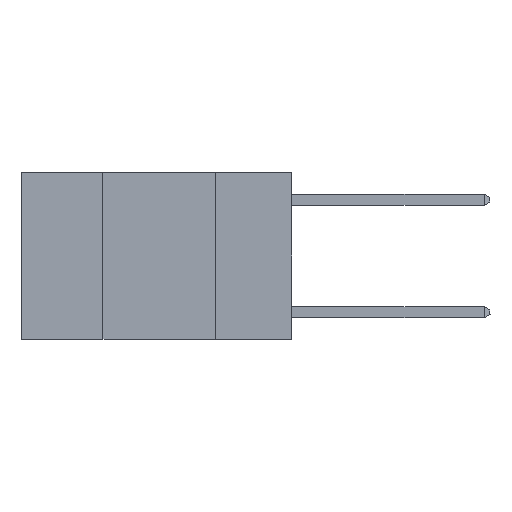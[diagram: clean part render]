
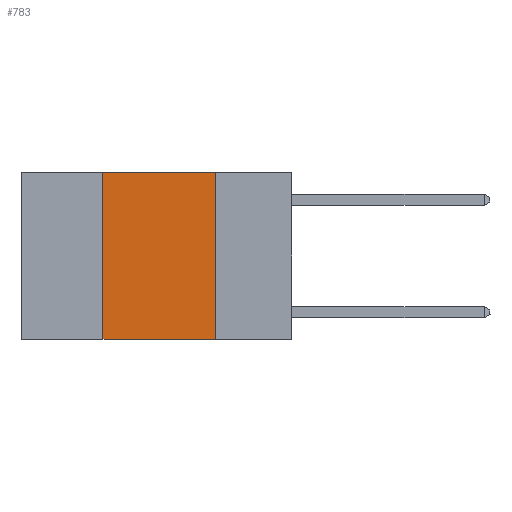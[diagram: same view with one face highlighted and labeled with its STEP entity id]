
A CAD part, left-side view. The second image highlights one B-rep face of the part: STEP entity #783.
In plain terms, the highlighted planar face has unit normal (-1, 0, 0).
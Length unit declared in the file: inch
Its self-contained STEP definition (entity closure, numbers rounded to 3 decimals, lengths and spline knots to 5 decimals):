
#232 = LINE ( 'NONE', #2339, #8810 ) ;
#305 = CARTESIAN_POINT ( 'NONE',  ( 0., 0.6, 0. ) ) ;
#434 = FACE_OUTER_BOUND ( 'NONE', #3041, .T. ) ;
#455 = VERTEX_POINT ( 'NONE', #8844 ) ;
#783 = ADVANCED_FACE ( 'NONE', ( #434 ), #3638, .F. ) ;
#1114 = ORIENTED_EDGE ( 'NONE', *, *, #6285, .F. ) ;
#1463 = ORIENTED_EDGE ( 'NONE', *, *, #6756, .F. ) ;
#1543 = DIRECTION ( 'NONE',  ( 0., 0., 1. ) ) ;
#1560 = VERTEX_POINT ( 'NONE', #4932 ) ;
#2214 = CARTESIAN_POINT ( 'NONE',  ( 0., 0.17, -0.37 ) ) ;
#2316 = CARTESIAN_POINT ( 'NONE',  ( 0., 0.17, 0. ) ) ;
#2339 = CARTESIAN_POINT ( 'NONE',  ( 0., 0.6, -0.37 ) ) ;
#3004 = VERTEX_POINT ( 'NONE', #2214 ) ;
#3041 = EDGE_LOOP ( 'NONE', ( #1114, #9660, #1463, #9987 ) ) ;
#3102 = LINE ( 'NONE', #8074, #5683 ) ;
#3232 = AXIS2_PLACEMENT_3D ( 'NONE', #10484, #10206, #11033 ) ;
#3422 = DIRECTION ( 'NONE',  ( 0., 0., -1. ) ) ;
#3638 = PLANE ( 'NONE',  #3232 ) ;
#4723 = LINE ( 'NONE', #2316, #6883 ) ;
#4932 = CARTESIAN_POINT ( 'NONE',  ( 0., 0.17, 0. ) ) ;
#5016 = VECTOR ( 'NONE', #7881, 39.37008 ) ;
#5339 = LINE ( 'NONE', #305, #5016 ) ;
#5683 = VECTOR ( 'NONE', #1543, 39.37008 ) ;
#6285 = EDGE_CURVE ( 'NONE', #1560, #3004, #4723, .T. ) ;
#6756 = EDGE_CURVE ( 'NONE', #455, #7239, #3102, .T. ) ;
#6883 = VECTOR ( 'NONE', #3422, 39.37008 ) ;
#7209 = EDGE_CURVE ( 'NONE', #455, #3004, #232, .T. ) ;
#7239 = VERTEX_POINT ( 'NONE', #7789 ) ;
#7283 = EDGE_CURVE ( 'NONE', #7239, #1560, #5339, .T. ) ;
#7789 = CARTESIAN_POINT ( 'NONE',  ( 0., 0.42, 0. ) ) ;
#7881 = DIRECTION ( 'NONE',  ( 0., -1., 0. ) ) ;
#8074 = CARTESIAN_POINT ( 'NONE',  ( 0., 0.42, 0. ) ) ;
#8810 = VECTOR ( 'NONE', #9805, 39.37008 ) ;
#8844 = CARTESIAN_POINT ( 'NONE',  ( 0., 0.42, -0.37 ) ) ;
#9660 = ORIENTED_EDGE ( 'NONE', *, *, #7283, .F. ) ;
#9805 = DIRECTION ( 'NONE',  ( 0., -1., 0. ) ) ;
#9987 = ORIENTED_EDGE ( 'NONE', *, *, #7209, .T. ) ;
#10206 = DIRECTION ( 'NONE',  ( 1., 0., 0. ) ) ;
#10484 = CARTESIAN_POINT ( 'NONE',  ( 0., 0.6, 0. ) ) ;
#11033 = DIRECTION ( 'NONE',  ( 0., 0., -1. ) ) ;
